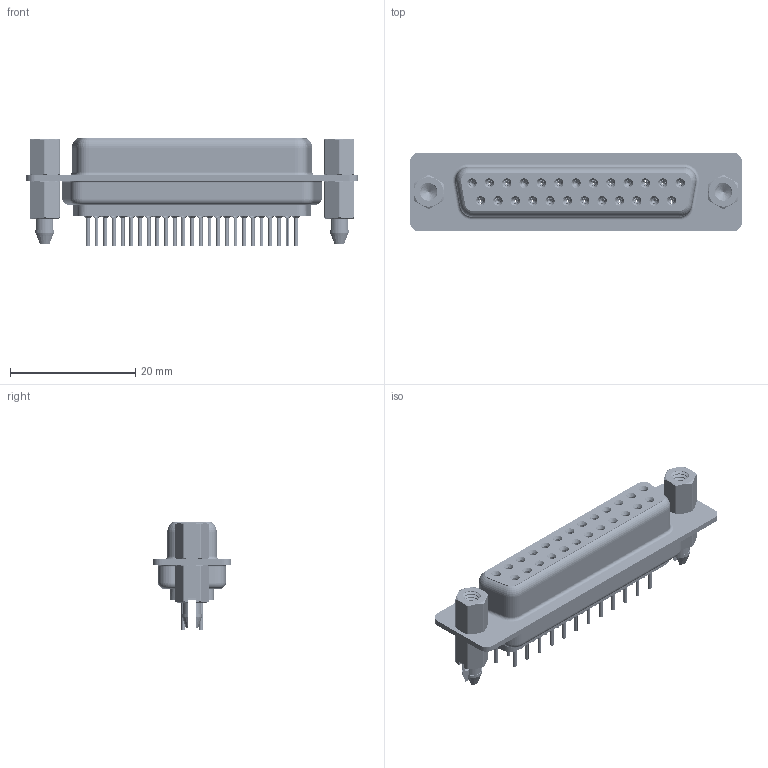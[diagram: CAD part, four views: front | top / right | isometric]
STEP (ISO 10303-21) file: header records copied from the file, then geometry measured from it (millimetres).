
FILE_DESCRIPTION (( 'STEP AP203' ), '1' );
FILE_NAME ('628-025-320-047.STEP', '2020-07-14T13:17:42', ( '' ), ( '' ), 'SwSTEP 2.0', 'SolidWorks 2020', '' );
FILE_SCHEMA (( 'CONFIG_CONTROL_DESIGN' ));
Length unit declared in the file: millimetre
Products named in the file (8): 628 Contact Row 2_20L; 628 4-40 Threaded Boardlock_LP; 628 Housing_25 LP; 628 Shell Front_25 Contacts; 628 4-40 Hex Standoff; 628-025-320-047; 628 Contact Row 1_20L; 628 Shell Rear_25 Contacts
Assembly tree (32 placements, depth 2):
  628-025-320-047
    628 Housing_25 LP
    628 Shell Front_25 Contacts
    628 Shell Rear_25 Contacts
    628 Contact Row 1_20L  x13
    628 Contact Row 2_20L  x12
    628 4-40 Hex Standoff  x2
    628 4-40 Threaded Boardlock_LP  x2
Bounding box: 53 x 12.6 x 17.3 mm (x, y, z)
Volume: 4163.5 mm3; surface area: 10117.3 mm2
Topology: 32 solids, 32 shells, 3654 faces, 9365 edges, 5834 vertices
Faces by surface type: cylinder 1066, plane 896, torus 713, bspline 518, cone 461
Entity records: 33836 total; most frequent: CARTESIAN_POINT 11318, DIRECTION 4525, ORIENTED_EDGE 4348, EDGE_CURVE 2174, AXIS2_PLACEMENT_3D 1878, VERTEX_POINT 1378, EDGE_LOOP 1044, CIRCLE 997
